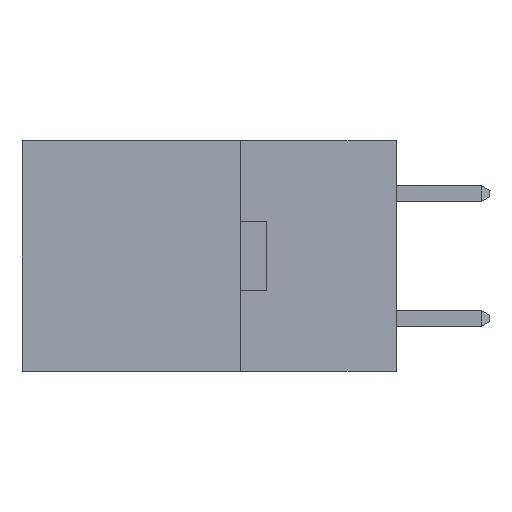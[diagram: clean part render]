
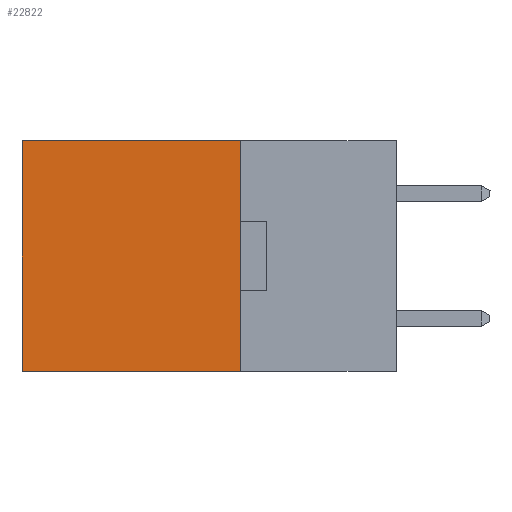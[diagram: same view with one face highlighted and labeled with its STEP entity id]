
A CAD part, left-side view. The second image highlights one B-rep face of the part: STEP entity #22822.
In plain terms, the highlighted planar face has unit normal (-1, 0, 0).
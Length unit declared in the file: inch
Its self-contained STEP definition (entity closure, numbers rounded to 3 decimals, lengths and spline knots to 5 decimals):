
#224 = DIRECTION ( 'NONE',  ( 0., 0., -1. ) ) ;
#1435 = DIRECTION ( 'NONE',  ( 0., 1., 0. ) ) ;
#3639 = LINE ( 'NONE', #25177, #14500 ) ;
#4141 = ORIENTED_EDGE ( 'NONE', *, *, #9851, .T. ) ;
#4830 = VERTEX_POINT ( 'NONE', #17926 ) ;
#5178 = LINE ( 'NONE', #9203, #8907 ) ;
#6355 = EDGE_CURVE ( 'NONE', #25720, #24411, #6384, .T. ) ;
#6384 = LINE ( 'NONE', #18677, #23423 ) ;
#6698 = VECTOR ( 'NONE', #10571, 39.37008 ) ;
#8868 = CARTESIAN_POINT ( 'NONE',  ( 0.2615, 0.25, -0.37 ) ) ;
#8907 = VECTOR ( 'NONE', #22060, 39.37008 ) ;
#9203 = CARTESIAN_POINT ( 'NONE',  ( 0.2615, 0.25, 0. ) ) ;
#9851 = EDGE_CURVE ( 'NONE', #13202, #4830, #5178, .T. ) ;
#10571 = DIRECTION ( 'NONE',  ( 0., 0., -1. ) ) ;
#11130 = ORIENTED_EDGE ( 'NONE', *, *, #23659, .T. ) ;
#13202 = VERTEX_POINT ( 'NONE', #25395 ) ;
#13227 = DIRECTION ( 'NONE',  ( 1., 0., 0. ) ) ;
#13298 = ORIENTED_EDGE ( 'NONE', *, *, #23747, .F. ) ;
#13854 = FACE_OUTER_BOUND ( 'NONE', #18425, .T. ) ;
#14500 = VECTOR ( 'NONE', #25257, 39.37008 ) ;
#17039 = CARTESIAN_POINT ( 'NONE',  ( 0.2615, 0.6, -0.37 ) ) ;
#17070 = CARTESIAN_POINT ( 'NONE',  ( 0.2615, 0.25, -0.37 ) ) ;
#17926 = CARTESIAN_POINT ( 'NONE',  ( 0.2615, 0.6, 0. ) ) ;
#18150 = LINE ( 'NONE', #17070, #6698 ) ;
#18425 = EDGE_LOOP ( 'NONE', ( #11130, #27653, #13298, #4141 ) ) ;
#18677 = CARTESIAN_POINT ( 'NONE',  ( 0.2615, 0.25, -0.37 ) ) ;
#19097 = AXIS2_PLACEMENT_3D ( 'NONE', #8868, #13227, #224 ) ;
#19191 = CARTESIAN_POINT ( 'NONE',  ( 0.2615, 0.25, -0.37 ) ) ;
#21633 = PLANE ( 'NONE',  #19097 ) ;
#22060 = DIRECTION ( 'NONE',  ( 0., 1., 0. ) ) ;
#22822 = ADVANCED_FACE ( 'NONE', ( #13854 ), #21633, .F. ) ;
#23423 = VECTOR ( 'NONE', #1435, 39.37008 ) ;
#23659 = EDGE_CURVE ( 'NONE', #4830, #24411, #3639, .T. ) ;
#23747 = EDGE_CURVE ( 'NONE', #13202, #25720, #18150, .T. ) ;
#24411 = VERTEX_POINT ( 'NONE', #17039 ) ;
#25177 = CARTESIAN_POINT ( 'NONE',  ( 0.2615, 0.6, -0.37 ) ) ;
#25257 = DIRECTION ( 'NONE',  ( 0., 0., -1. ) ) ;
#25395 = CARTESIAN_POINT ( 'NONE',  ( 0.2615, 0.25, 0. ) ) ;
#25720 = VERTEX_POINT ( 'NONE', #19191 ) ;
#27653 = ORIENTED_EDGE ( 'NONE', *, *, #6355, .F. ) ;
